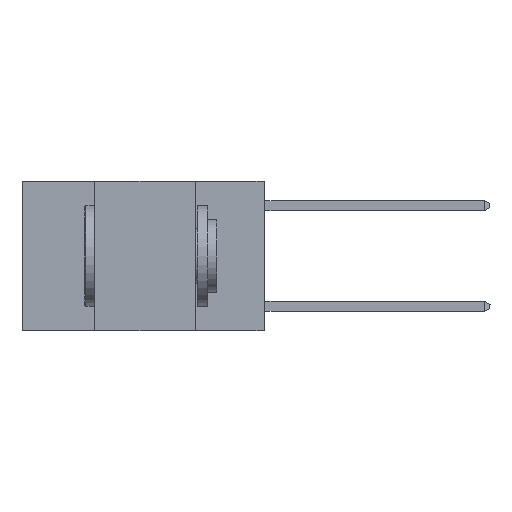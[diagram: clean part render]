
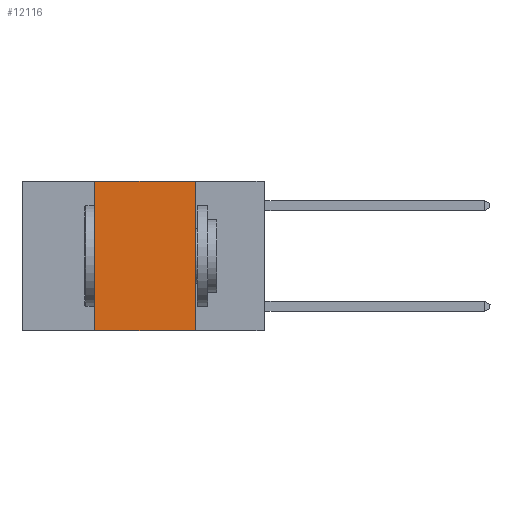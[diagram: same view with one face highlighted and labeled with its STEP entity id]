
A CAD part, left-side view. The second image highlights one B-rep face of the part: STEP entity #12116.
In plain terms, the highlighted planar face has unit normal (-1, 0, 0).
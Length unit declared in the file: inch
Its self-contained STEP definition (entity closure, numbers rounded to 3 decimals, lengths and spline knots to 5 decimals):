
#151 = VERTEX_POINT ( 'NONE', #1609 ) ;
#429 = LINE ( 'NONE', #11229, #11002 ) ;
#1221 = FACE_OUTER_BOUND ( 'NONE', #5104, .T. ) ;
#1402 = VECTOR ( 'NONE', #13010, 39.37008 ) ;
#1503 = ORIENTED_EDGE ( 'NONE', *, *, #10991, .F. ) ;
#1609 = CARTESIAN_POINT ( 'NONE',  ( 0., 0.17, 0. ) ) ;
#2230 = DIRECTION ( 'NONE',  ( 0., -1., 0. ) ) ;
#2322 = VECTOR ( 'NONE', #2230, 39.37008 ) ;
#2660 = LINE ( 'NONE', #11426, #2322 ) ;
#3041 = DIRECTION ( 'NONE',  ( 0., 0., -1. ) ) ;
#3533 = LINE ( 'NONE', #12149, #5958 ) ;
#4156 = DIRECTION ( 'NONE',  ( 0., 0., -1. ) ) ;
#4231 = CARTESIAN_POINT ( 'NONE',  ( 0., 0.42, 0. ) ) ;
#5104 = EDGE_LOOP ( 'NONE', ( #1503, #9668, #12648, #10322 ) ) ;
#5115 = VERTEX_POINT ( 'NONE', #4231 ) ;
#5958 = VECTOR ( 'NONE', #3041, 39.37008 ) ;
#6224 = EDGE_CURVE ( 'NONE', #5115, #151, #8949, .T. ) ;
#6763 = CARTESIAN_POINT ( 'NONE',  ( 0., 0.17, -0.37 ) ) ;
#7209 = CARTESIAN_POINT ( 'NONE',  ( 0., 0.42, -0.37 ) ) ;
#7236 = DIRECTION ( 'NONE',  ( 0., 0., 1. ) ) ;
#7535 = EDGE_CURVE ( 'NONE', #11003, #11249, #2660, .T. ) ;
#8216 = CARTESIAN_POINT ( 'NONE',  ( 0., 0.6, 0. ) ) ;
#8510 = AXIS2_PLACEMENT_3D ( 'NONE', #8216, #10242, #4156 ) ;
#8949 = LINE ( 'NONE', #8982, #1402 ) ;
#8982 = CARTESIAN_POINT ( 'NONE',  ( 0., 0.6, 0. ) ) ;
#9235 = PLANE ( 'NONE',  #8510 ) ;
#9668 = ORIENTED_EDGE ( 'NONE', *, *, #6224, .F. ) ;
#10242 = DIRECTION ( 'NONE',  ( 1., 0., 0. ) ) ;
#10322 = ORIENTED_EDGE ( 'NONE', *, *, #7535, .T. ) ;
#10991 = EDGE_CURVE ( 'NONE', #151, #11249, #3533, .T. ) ;
#11002 = VECTOR ( 'NONE', #7236, 39.37008 ) ;
#11003 = VERTEX_POINT ( 'NONE', #7209 ) ;
#11229 = CARTESIAN_POINT ( 'NONE',  ( 0., 0.42, 0. ) ) ;
#11249 = VERTEX_POINT ( 'NONE', #6763 ) ;
#11426 = CARTESIAN_POINT ( 'NONE',  ( 0., 0.6, -0.37 ) ) ;
#11490 = EDGE_CURVE ( 'NONE', #11003, #5115, #429, .T. ) ;
#12116 = ADVANCED_FACE ( 'NONE', ( #1221 ), #9235, .F. ) ;
#12149 = CARTESIAN_POINT ( 'NONE',  ( 0., 0.17, 0. ) ) ;
#12648 = ORIENTED_EDGE ( 'NONE', *, *, #11490, .F. ) ;
#13010 = DIRECTION ( 'NONE',  ( 0., -1., 0. ) ) ;
